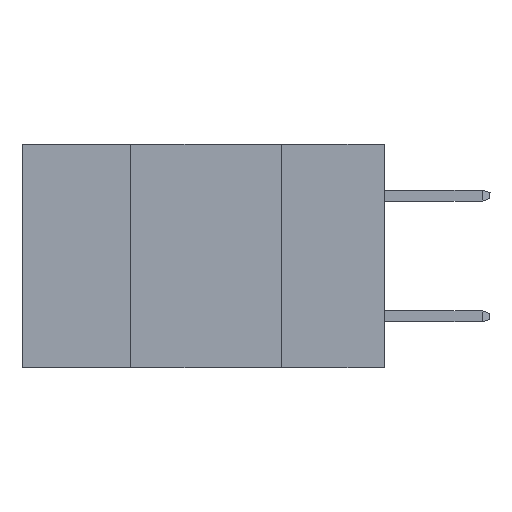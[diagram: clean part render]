
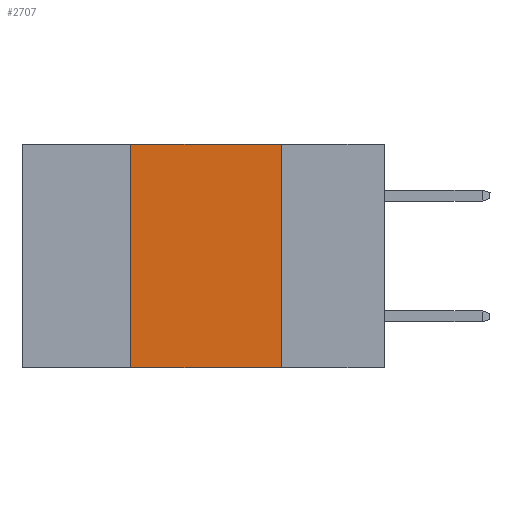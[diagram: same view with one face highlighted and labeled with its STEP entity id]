
A CAD part, left-side view. The second image highlights one B-rep face of the part: STEP entity #2707.
In plain terms, the highlighted planar face has unit normal (-1, 0, 0).
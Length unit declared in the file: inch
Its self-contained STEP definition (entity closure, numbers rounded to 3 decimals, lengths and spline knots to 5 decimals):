
#411 = LINE ( 'NONE', #15642, #8492 ) ;
#816 = CARTESIAN_POINT ( 'NONE',  ( 0., 0.6, 0. ) ) ;
#842 = DIRECTION ( 'NONE',  ( 0., -1., 0. ) ) ;
#884 = CARTESIAN_POINT ( 'NONE',  ( 0., 0.42, 0. ) ) ;
#939 = CARTESIAN_POINT ( 'NONE',  ( 0., 0.6, 0. ) ) ;
#1176 = LINE ( 'NONE', #884, #12335 ) ;
#1366 = VERTEX_POINT ( 'NONE', #4301 ) ;
#1814 = VERTEX_POINT ( 'NONE', #11450 ) ;
#2707 = ADVANCED_FACE ( 'NONE', ( #11459 ), #15495, .F. ) ;
#3315 = DIRECTION ( 'NONE',  ( 0., 0., -1. ) ) ;
#4212 = LINE ( 'NONE', #15517, #13979 ) ;
#4279 = AXIS2_PLACEMENT_3D ( 'NONE', #816, #14301, #3315 ) ;
#4301 = CARTESIAN_POINT ( 'NONE',  ( 0., 0.17, 0. ) ) ;
#4306 = EDGE_CURVE ( 'NONE', #1366, #10256, #411, .T. ) ;
#4670 = DIRECTION ( 'NONE',  ( 0., 0., -1. ) ) ;
#5660 = DIRECTION ( 'NONE',  ( 0., 0., 1. ) ) ;
#8073 = EDGE_CURVE ( 'NONE', #1814, #1366, #12587, .T. ) ;
#8469 = ORIENTED_EDGE ( 'NONE', *, *, #4306, .F. ) ;
#8492 = VECTOR ( 'NONE', #4670, 39.37008 ) ;
#9079 = CARTESIAN_POINT ( 'NONE',  ( 0., 0.42, -0.37 ) ) ;
#9192 = EDGE_CURVE ( 'NONE', #14965, #1814, #1176, .T. ) ;
#9356 = ORIENTED_EDGE ( 'NONE', *, *, #8073, .F. ) ;
#9384 = EDGE_LOOP ( 'NONE', ( #8469, #9356, #12585, #12229 ) ) ;
#10256 = VERTEX_POINT ( 'NONE', #14602 ) ;
#10280 = VECTOR ( 'NONE', #13293, 39.37008 ) ;
#11354 = EDGE_CURVE ( 'NONE', #14965, #10256, #4212, .T. ) ;
#11450 = CARTESIAN_POINT ( 'NONE',  ( 0., 0.42, 0. ) ) ;
#11459 = FACE_OUTER_BOUND ( 'NONE', #9384, .T. ) ;
#12229 = ORIENTED_EDGE ( 'NONE', *, *, #11354, .T. ) ;
#12335 = VECTOR ( 'NONE', #5660, 39.37008 ) ;
#12585 = ORIENTED_EDGE ( 'NONE', *, *, #9192, .F. ) ;
#12587 = LINE ( 'NONE', #939, #10280 ) ;
#13293 = DIRECTION ( 'NONE',  ( 0., -1., 0. ) ) ;
#13979 = VECTOR ( 'NONE', #842, 39.37008 ) ;
#14301 = DIRECTION ( 'NONE',  ( 1., 0., 0. ) ) ;
#14602 = CARTESIAN_POINT ( 'NONE',  ( 0., 0.17, -0.37 ) ) ;
#14965 = VERTEX_POINT ( 'NONE', #9079 ) ;
#15495 = PLANE ( 'NONE',  #4279 ) ;
#15517 = CARTESIAN_POINT ( 'NONE',  ( 0., 0.6, -0.37 ) ) ;
#15642 = CARTESIAN_POINT ( 'NONE',  ( 0., 0.17, 0. ) ) ;
